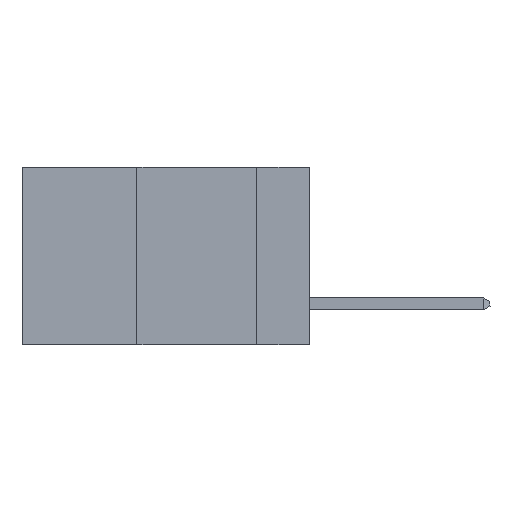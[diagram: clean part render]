
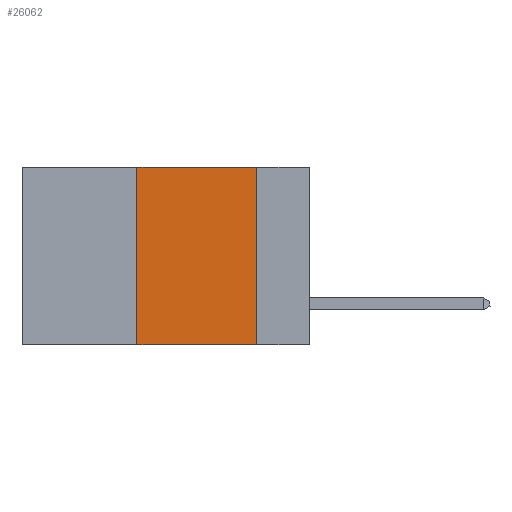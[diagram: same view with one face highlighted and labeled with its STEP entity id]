
A CAD part, left-side view. The second image highlights one B-rep face of the part: STEP entity #26062.
In plain terms, the highlighted planar face has unit normal (-1, 0, 0).
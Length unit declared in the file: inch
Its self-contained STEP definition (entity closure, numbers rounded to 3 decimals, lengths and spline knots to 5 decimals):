
#44 = VERTEX_POINT ( 'NONE', #18877 ) ;
#209 = ORIENTED_EDGE ( 'NONE', *, *, #5050, .F. ) ;
#1022 = CARTESIAN_POINT ( 'NONE',  ( 0., 0.36, 0. ) ) ;
#1518 = ORIENTED_EDGE ( 'NONE', *, *, #5335, .F. ) ;
#1673 = EDGE_LOOP ( 'NONE', ( #209, #1518, #9069, #12983 ) ) ;
#2786 = VECTOR ( 'NONE', #24970, 39.37008 ) ;
#3096 = DIRECTION ( 'NONE',  ( 0., 0., 1. ) ) ;
#3432 = LINE ( 'NONE', #1022, #24808 ) ;
#3520 = CARTESIAN_POINT ( 'NONE',  ( 0., 0.11, 0. ) ) ;
#3645 = DIRECTION ( 'NONE',  ( 0., 0., -1. ) ) ;
#4401 = VECTOR ( 'NONE', #5632, 39.37008 ) ;
#4893 = EDGE_CURVE ( 'NONE', #44, #6577, #3432, .T. ) ;
#5050 = EDGE_CURVE ( 'NONE', #13333, #5582, #20933, .T. ) ;
#5335 = EDGE_CURVE ( 'NONE', #6577, #13333, #19319, .T. ) ;
#5582 = VERTEX_POINT ( 'NONE', #7191 ) ;
#5632 = DIRECTION ( 'NONE',  ( 0., 0., -1. ) ) ;
#6577 = VERTEX_POINT ( 'NONE', #13428 ) ;
#7191 = CARTESIAN_POINT ( 'NONE',  ( 0., 0.11, -0.37 ) ) ;
#7941 = AXIS2_PLACEMENT_3D ( 'NONE', #14091, #16165, #3645 ) ;
#8500 = CARTESIAN_POINT ( 'NONE',  ( 0., 0.6, 0. ) ) ;
#9069 = ORIENTED_EDGE ( 'NONE', *, *, #4893, .F. ) ;
#11168 = CARTESIAN_POINT ( 'NONE',  ( 0., 0.11, 0. ) ) ;
#12982 = EDGE_CURVE ( 'NONE', #44, #5582, #13688, .T. ) ;
#12983 = ORIENTED_EDGE ( 'NONE', *, *, #12982, .T. ) ;
#13333 = VERTEX_POINT ( 'NONE', #11168 ) ;
#13428 = CARTESIAN_POINT ( 'NONE',  ( 0., 0.36, 0. ) ) ;
#13688 = LINE ( 'NONE', #26413, #18475 ) ;
#14091 = CARTESIAN_POINT ( 'NONE',  ( 0., 0.6, 0. ) ) ;
#16165 = DIRECTION ( 'NONE',  ( 1., 0., 0. ) ) ;
#17322 = FACE_OUTER_BOUND ( 'NONE', #1673, .T. ) ;
#18259 = DIRECTION ( 'NONE',  ( 0., -1., 0. ) ) ;
#18475 = VECTOR ( 'NONE', #18259, 39.37008 ) ;
#18877 = CARTESIAN_POINT ( 'NONE',  ( 0., 0.36, -0.37 ) ) ;
#19319 = LINE ( 'NONE', #8500, #2786 ) ;
#20933 = LINE ( 'NONE', #3520, #4401 ) ;
#24808 = VECTOR ( 'NONE', #3096, 39.37008 ) ;
#24970 = DIRECTION ( 'NONE',  ( 0., -1., 0. ) ) ;
#26062 = ADVANCED_FACE ( 'NONE', ( #17322 ), #26355, .F. ) ;
#26355 = PLANE ( 'NONE',  #7941 ) ;
#26413 = CARTESIAN_POINT ( 'NONE',  ( 0., 0.6, -0.37 ) ) ;
